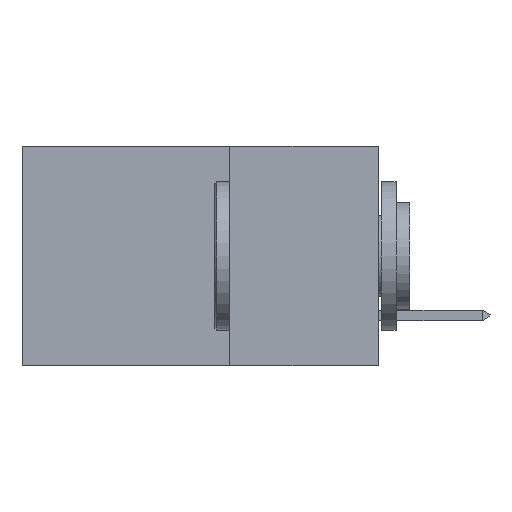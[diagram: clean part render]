
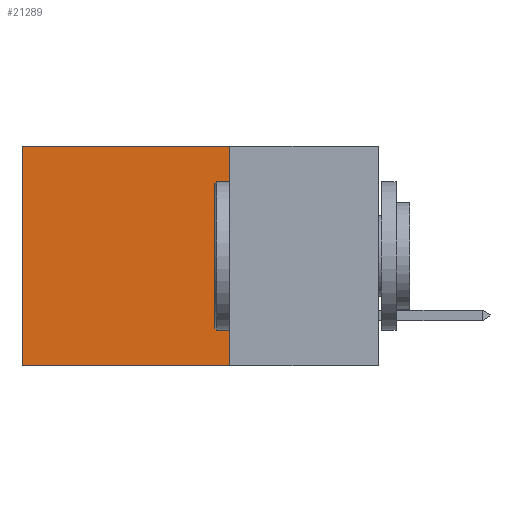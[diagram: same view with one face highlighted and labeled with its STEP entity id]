
A CAD part, left-side view. The second image highlights one B-rep face of the part: STEP entity #21289.
In plain terms, the highlighted planar face has unit normal (-1, 0, 0).
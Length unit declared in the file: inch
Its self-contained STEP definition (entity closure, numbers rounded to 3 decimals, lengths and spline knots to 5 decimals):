
#273 = LINE ( 'NONE', #9498, #24766 ) ;
#330 = DIRECTION ( 'NONE',  ( 0., 0., -1. ) ) ;
#528 = EDGE_CURVE ( 'NONE', #25578, #23716, #20144, .T. ) ;
#894 = FACE_OUTER_BOUND ( 'NONE', #6848, .T. ) ;
#2542 = ORIENTED_EDGE ( 'NONE', *, *, #21607, .T. ) ;
#3277 = CARTESIAN_POINT ( 'NONE',  ( 0.298, 0.25, 0. ) ) ;
#4209 = DIRECTION ( 'NONE',  ( 0., 1., 0. ) ) ;
#5676 = VECTOR ( 'NONE', #13237, 39.37008 ) ;
#6848 = EDGE_LOOP ( 'NONE', ( #23470, #24564, #20241, #2542 ) ) ;
#6868 = LINE ( 'NONE', #18411, #25020 ) ;
#7735 = EDGE_CURVE ( 'NONE', #23716, #26871, #30536, .T. ) ;
#9498 = CARTESIAN_POINT ( 'NONE',  ( 0.298, 0.6, 0. ) ) ;
#11225 = AXIS2_PLACEMENT_3D ( 'NONE', #3277, #14986, #21853 ) ;
#12849 = PLANE ( 'NONE',  #11225 ) ;
#13237 = DIRECTION ( 'NONE',  ( 0., 0., -1. ) ) ;
#13776 = CARTESIAN_POINT ( 'NONE',  ( 0.298, 0.25, 0. ) ) ;
#14986 = DIRECTION ( 'NONE',  ( 1., 0., 0. ) ) ;
#16066 = CARTESIAN_POINT ( 'NONE',  ( 0.298, 0.6, -0.37 ) ) ;
#18059 = VERTEX_POINT ( 'NONE', #22669 ) ;
#18411 = CARTESIAN_POINT ( 'NONE',  ( 0.298, 0.25, 0. ) ) ;
#20144 = LINE ( 'NONE', #27443, #5676 ) ;
#20241 = ORIENTED_EDGE ( 'NONE', *, *, #528, .F. ) ;
#20602 = EDGE_CURVE ( 'NONE', #18059, #26871, #273, .T. ) ;
#21289 = ADVANCED_FACE ( 'NONE', ( #894 ), #12849, .F. ) ;
#21607 = EDGE_CURVE ( 'NONE', #25578, #18059, #6868, .T. ) ;
#21621 = CARTESIAN_POINT ( 'NONE',  ( 0.298, 0.25, -0.37 ) ) ;
#21853 = DIRECTION ( 'NONE',  ( 0., 0., -1. ) ) ;
#22669 = CARTESIAN_POINT ( 'NONE',  ( 0.298, 0.6, 0. ) ) ;
#22800 = CARTESIAN_POINT ( 'NONE',  ( 0.298, 0.25, -0.37 ) ) ;
#23470 = ORIENTED_EDGE ( 'NONE', *, *, #20602, .T. ) ;
#23716 = VERTEX_POINT ( 'NONE', #22800 ) ;
#24564 = ORIENTED_EDGE ( 'NONE', *, *, #7735, .F. ) ;
#24766 = VECTOR ( 'NONE', #330, 39.37008 ) ;
#25020 = VECTOR ( 'NONE', #4209, 39.37008 ) ;
#25578 = VERTEX_POINT ( 'NONE', #13776 ) ;
#26108 = VECTOR ( 'NONE', #27777, 39.37008 ) ;
#26871 = VERTEX_POINT ( 'NONE', #16066 ) ;
#27443 = CARTESIAN_POINT ( 'NONE',  ( 0.298, 0.25, 0. ) ) ;
#27777 = DIRECTION ( 'NONE',  ( 0., 1., 0. ) ) ;
#30536 = LINE ( 'NONE', #21621, #26108 ) ;
